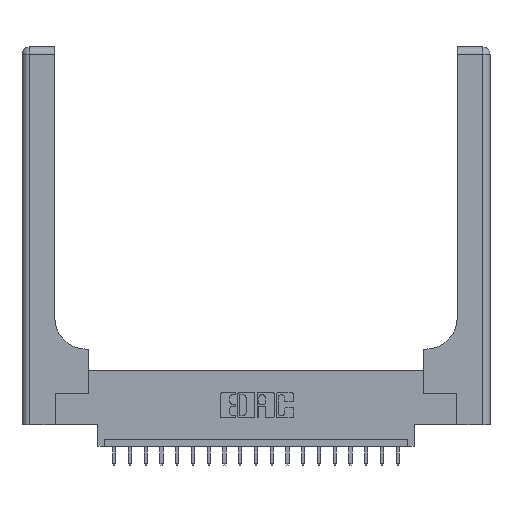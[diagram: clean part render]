
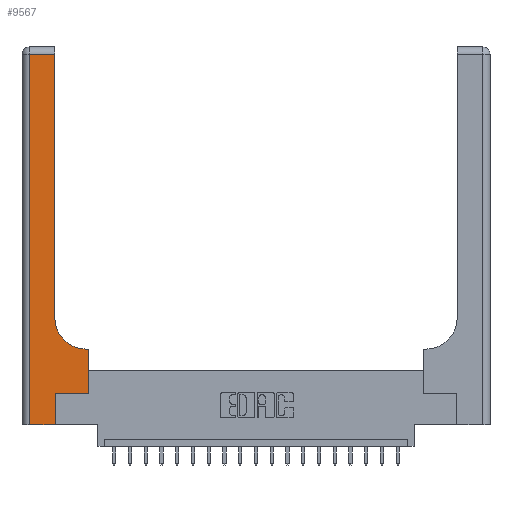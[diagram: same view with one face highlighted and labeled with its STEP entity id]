
A CAD part, top view. The second image highlights one B-rep face of the part: STEP entity #9567.
In plain terms, the highlighted planar face has unit normal (0, 0, 1).
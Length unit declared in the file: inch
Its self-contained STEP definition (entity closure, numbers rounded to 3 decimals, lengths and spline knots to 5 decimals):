
#26 = VERTEX_POINT ( 'NONE', #12949 ) ;
#464 = ORIENTED_EDGE ( 'NONE', *, *, #16489, .T. ) ;
#627 = LINE ( 'NONE', #13480, #5927 ) ;
#742 = FACE_OUTER_BOUND ( 'NONE', #3592, .T. ) ;
#913 = CIRCLE ( 'NONE', #10573, 0.25 ) ;
#1063 = ORIENTED_EDGE ( 'NONE', *, *, #7733, .T. ) ;
#1259 = VERTEX_POINT ( 'NONE', #2480 ) ;
#1840 = VECTOR ( 'NONE', #2331, 39.37008 ) ;
#2147 = DIRECTION ( 'NONE',  ( -1., 0., 0. ) ) ;
#2323 = ORIENTED_EDGE ( 'NONE', *, *, #12842, .T. ) ;
#2331 = DIRECTION ( 'NONE',  ( 0., -1., 0. ) ) ;
#2480 = CARTESIAN_POINT ( 'NONE',  ( 0.06, 2.94, 0.37 ) ) ;
#2483 = ORIENTED_EDGE ( 'NONE', *, *, #3686, .T. ) ;
#3113 = DIRECTION ( 'NONE',  ( 1., 0., 0. ) ) ;
#3308 = CARTESIAN_POINT ( 'NONE',  ( 0., 3., 0.37 ) ) ;
#3363 = LINE ( 'NONE', #6504, #15985 ) ;
#3382 = LINE ( 'NONE', #13212, #17700 ) ;
#3592 = EDGE_LOOP ( 'NONE', ( #2483, #8244, #8469, #464, #7132, #15447, #1063, #10347, #2323 ) ) ;
#3645 = CARTESIAN_POINT ( 'NONE',  ( 0.528, 0.25, 0.37 ) ) ;
#3686 = EDGE_CURVE ( 'NONE', #12852, #18724, #627, .T. ) ;
#3862 = LINE ( 'NONE', #6619, #10932 ) ;
#4362 = CARTESIAN_POINT ( 'NONE',  ( 0.26, 0.85, 0.37 ) ) ;
#4718 = EDGE_CURVE ( 'NONE', #1259, #10211, #18437, .T. ) ;
#4756 = LINE ( 'NONE', #18881, #13041 ) ;
#5100 = VECTOR ( 'NONE', #2147, 39.37008 ) ;
#5196 = DIRECTION ( 'NONE',  ( 1., 0., 0. ) ) ;
#5414 = AXIS2_PLACEMENT_3D ( 'NONE', #3308, #17639, #14397 ) ;
#5736 = EDGE_CURVE ( 'NONE', #18724, #1259, #8304, .T. ) ;
#5927 = VECTOR ( 'NONE', #6993, 39.37008 ) ;
#5935 = VERTEX_POINT ( 'NONE', #7450 ) ;
#6504 = CARTESIAN_POINT ( 'NONE',  ( 0.265, 0., 0.37 ) ) ;
#6619 = CARTESIAN_POINT ( 'NONE',  ( 0.528, 0.25, 0.37 ) ) ;
#6993 = DIRECTION ( 'NONE',  ( 0., 1., 0. ) ) ;
#7132 = ORIENTED_EDGE ( 'NONE', *, *, #14744, .T. ) ;
#7450 = CARTESIAN_POINT ( 'NONE',  ( 0.528, 0.6, 0.37 ) ) ;
#7637 = VECTOR ( 'NONE', #5196, 39.37008 ) ;
#7733 = EDGE_CURVE ( 'NONE', #11393, #5935, #3862, .T. ) ;
#8244 = ORIENTED_EDGE ( 'NONE', *, *, #5736, .T. ) ;
#8304 = LINE ( 'NONE', #16255, #5100 ) ;
#8466 = CARTESIAN_POINT ( 'NONE',  ( 0.51, 0.6, 0.37 ) ) ;
#8469 = ORIENTED_EDGE ( 'NONE', *, *, #4718, .T. ) ;
#8877 = EDGE_CURVE ( 'NONE', #26, #11393, #3382, .T. ) ;
#9414 = VERTEX_POINT ( 'NONE', #8466 ) ;
#9567 = ADVANCED_FACE ( 'NONE', ( #742 ), #10857, .F. ) ;
#10211 = VERTEX_POINT ( 'NONE', #16856 ) ;
#10253 = VERTEX_POINT ( 'NONE', #13635 ) ;
#10347 = ORIENTED_EDGE ( 'NONE', *, *, #18095, .T. ) ;
#10573 = AXIS2_PLACEMENT_3D ( 'NONE', #11152, #12309, #3113 ) ;
#10857 = PLANE ( 'NONE',  #5414 ) ;
#10932 = VECTOR ( 'NONE', #18297, 39.37008 ) ;
#11152 = CARTESIAN_POINT ( 'NONE',  ( 0.51, 0.85, 0.37 ) ) ;
#11393 = VERTEX_POINT ( 'NONE', #3645 ) ;
#11568 = CARTESIAN_POINT ( 'NONE',  ( 0., 0., 0.37 ) ) ;
#12309 = DIRECTION ( 'NONE',  ( 0., 0., -1. ) ) ;
#12842 = EDGE_CURVE ( 'NONE', #9414, #12852, #913, .T. ) ;
#12852 = VERTEX_POINT ( 'NONE', #4362 ) ;
#12949 = CARTESIAN_POINT ( 'NONE',  ( 0.265, 0.25, 0.37 ) ) ;
#13041 = VECTOR ( 'NONE', #17315, 39.37008 ) ;
#13212 = CARTESIAN_POINT ( 'NONE',  ( 0.265, 0.25, 0.37 ) ) ;
#13480 = CARTESIAN_POINT ( 'NONE',  ( 0.26, 3., 0.37 ) ) ;
#13635 = CARTESIAN_POINT ( 'NONE',  ( 0.265, 0., 0.37 ) ) ;
#14397 = DIRECTION ( 'NONE',  ( -1., 0., 0. ) ) ;
#14744 = EDGE_CURVE ( 'NONE', #10253, #26, #3363, .T. ) ;
#14774 = DIRECTION ( 'NONE',  ( 1., 0., 0. ) ) ;
#15285 = CARTESIAN_POINT ( 'NONE',  ( 0.26, 2.94, 0.37 ) ) ;
#15447 = ORIENTED_EDGE ( 'NONE', *, *, #8877, .T. ) ;
#15985 = VECTOR ( 'NONE', #19366, 39.37008 ) ;
#16255 = CARTESIAN_POINT ( 'NONE',  ( 0., 2.94, 0.37 ) ) ;
#16489 = EDGE_CURVE ( 'NONE', #10211, #10253, #17648, .T. ) ;
#16856 = CARTESIAN_POINT ( 'NONE',  ( 0.06, 0., 0.37 ) ) ;
#17315 = DIRECTION ( 'NONE',  ( -1., 0., 0. ) ) ;
#17639 = DIRECTION ( 'NONE',  ( 0., 0., -1. ) ) ;
#17648 = LINE ( 'NONE', #11568, #7637 ) ;
#17700 = VECTOR ( 'NONE', #14774, 39.37008 ) ;
#18095 = EDGE_CURVE ( 'NONE', #5935, #9414, #4756, .T. ) ;
#18240 = CARTESIAN_POINT ( 'NONE',  ( 0.06, 3., 0.37 ) ) ;
#18297 = DIRECTION ( 'NONE',  ( 0., 1., 0. ) ) ;
#18437 = LINE ( 'NONE', #18240, #1840 ) ;
#18724 = VERTEX_POINT ( 'NONE', #15285 ) ;
#18881 = CARTESIAN_POINT ( 'NONE',  ( 0.26, 0.6, 0.37 ) ) ;
#19366 = DIRECTION ( 'NONE',  ( 0., 1., 0. ) ) ;
